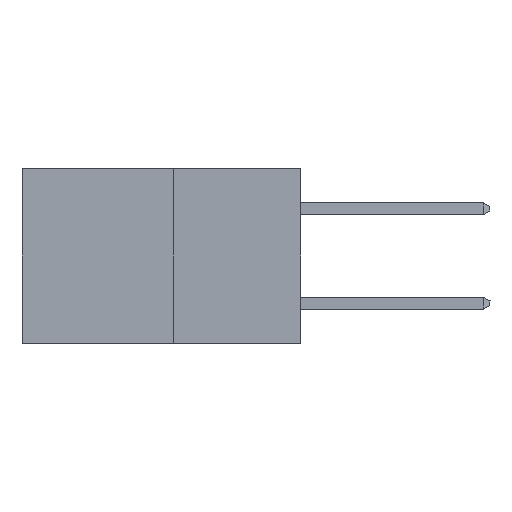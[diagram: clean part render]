
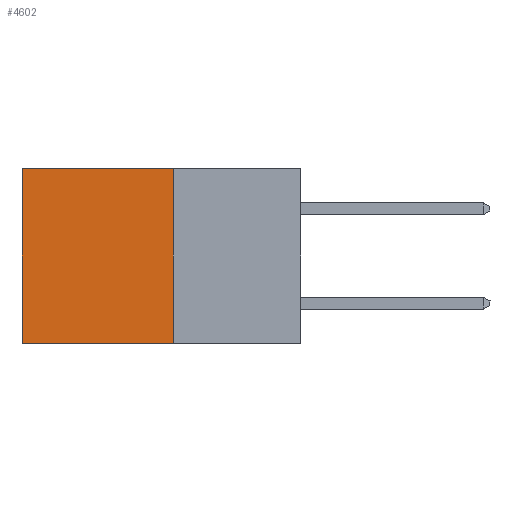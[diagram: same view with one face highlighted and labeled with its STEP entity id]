
A CAD part, left-side view. The second image highlights one B-rep face of the part: STEP entity #4602.
In plain terms, the highlighted planar face has unit normal (-1, 0, 0).
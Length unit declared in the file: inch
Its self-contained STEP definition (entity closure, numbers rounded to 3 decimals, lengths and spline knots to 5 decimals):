
#463 = CARTESIAN_POINT ( 'NONE',  ( 0.277, 0.27, -0.37 ) ) ;
#793 = ORIENTED_EDGE ( 'NONE', *, *, #6362, .T. ) ;
#912 = DIRECTION ( 'NONE',  ( 0., 0., -1. ) ) ;
#927 = DIRECTION ( 'NONE',  ( 1., 0., 0. ) ) ;
#1171 = VERTEX_POINT ( 'NONE', #4613 ) ;
#1176 = ORIENTED_EDGE ( 'NONE', *, *, #6950, .F. ) ;
#1444 = CARTESIAN_POINT ( 'NONE',  ( 0.277, 0.27, 0. ) ) ;
#1835 = VERTEX_POINT ( 'NONE', #6826 ) ;
#1984 = PLANE ( 'NONE',  #4736 ) ;
#1990 = LINE ( 'NONE', #2920, #6636 ) ;
#2137 = VECTOR ( 'NONE', #10801, 39.37008 ) ;
#2255 = CARTESIAN_POINT ( 'NONE',  ( 0.277, 0.27, -0.37 ) ) ;
#2914 = VECTOR ( 'NONE', #3813, 39.37008 ) ;
#2920 = CARTESIAN_POINT ( 'NONE',  ( 0.277, 0.59, -0.37 ) ) ;
#3813 = DIRECTION ( 'NONE',  ( 0., 0., -1. ) ) ;
#4185 = LINE ( 'NONE', #9826, #10903 ) ;
#4431 = LINE ( 'NONE', #2255, #2137 ) ;
#4602 = ADVANCED_FACE ( 'NONE', ( #4727 ), #1984, .F. ) ;
#4613 = CARTESIAN_POINT ( 'NONE',  ( 0.277, 0.59, -0.37 ) ) ;
#4628 = VERTEX_POINT ( 'NONE', #1444 ) ;
#4727 = FACE_OUTER_BOUND ( 'NONE', #10392, .T. ) ;
#4736 = AXIS2_PLACEMENT_3D ( 'NONE', #463, #927, #912 ) ;
#5212 = LINE ( 'NONE', #6957, #2914 ) ;
#5387 = CARTESIAN_POINT ( 'NONE',  ( 0.277, 0.59, 0. ) ) ;
#5594 = EDGE_CURVE ( 'NONE', #1835, #1171, #4431, .T. ) ;
#6092 = ORIENTED_EDGE ( 'NONE', *, *, #5594, .F. ) ;
#6362 = EDGE_CURVE ( 'NONE', #10762, #1171, #1990, .T. ) ;
#6459 = ORIENTED_EDGE ( 'NONE', *, *, #9495, .T. ) ;
#6636 = VECTOR ( 'NONE', #7275, 39.37008 ) ;
#6826 = CARTESIAN_POINT ( 'NONE',  ( 0.277, 0.27, -0.37 ) ) ;
#6950 = EDGE_CURVE ( 'NONE', #4628, #1835, #5212, .T. ) ;
#6957 = CARTESIAN_POINT ( 'NONE',  ( 0.277, 0.27, -0.37 ) ) ;
#7275 = DIRECTION ( 'NONE',  ( 0., 0., -1. ) ) ;
#9489 = DIRECTION ( 'NONE',  ( 0., 1., 0. ) ) ;
#9495 = EDGE_CURVE ( 'NONE', #4628, #10762, #4185, .T. ) ;
#9826 = CARTESIAN_POINT ( 'NONE',  ( 0.277, 0.27, 0. ) ) ;
#10392 = EDGE_LOOP ( 'NONE', ( #793, #6092, #1176, #6459 ) ) ;
#10762 = VERTEX_POINT ( 'NONE', #5387 ) ;
#10801 = DIRECTION ( 'NONE',  ( 0., 1., 0. ) ) ;
#10903 = VECTOR ( 'NONE', #9489, 39.37008 ) ;
